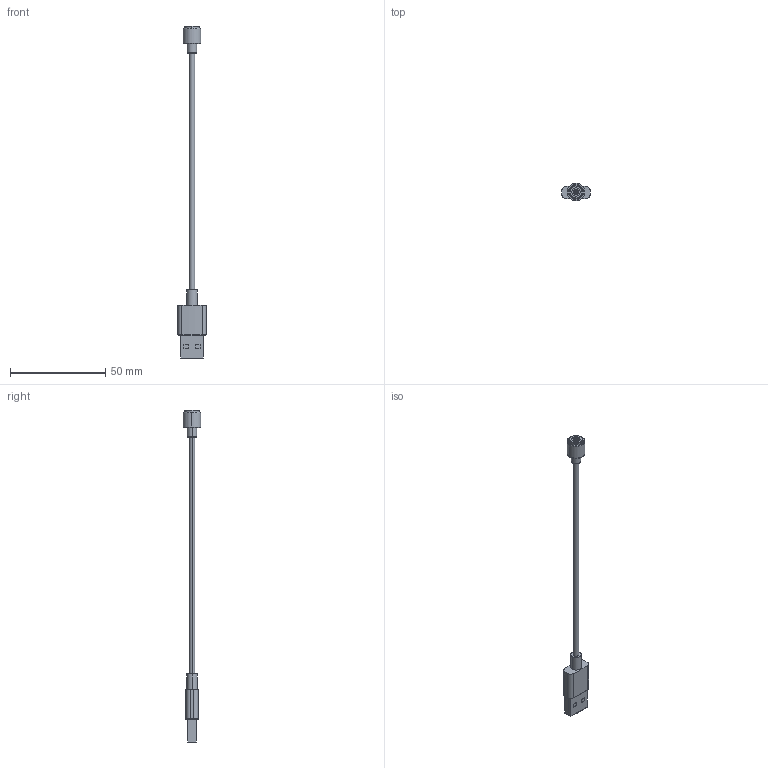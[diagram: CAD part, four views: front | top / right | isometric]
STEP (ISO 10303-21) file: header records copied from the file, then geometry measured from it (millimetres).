
FILE_DESCRIPTION (( 'STEP AP203' ), '1' );
FILE_NAME ('687-C0222A001C00.STEP', '2023-02-09T15:45:17', ( '' ), ( '' ), 'SwSTEP 2.0', 'SolidWorks 2020', '' );
FILE_SCHEMA (( 'CONFIG_CONTROL_DESIGN' ));
Length unit declared in the file: millimetre
Products named in the file (1): 687-C0222A001C00
Bounding box: 14.8 x 9.4 x 174.69 mm (x, y, z)
Surface area: 3758.1 mm2 (no closed solid volume)
Topology: 0 solids, 5 shells, 143 faces, 332 edges, 212 vertices
Faces by surface type: plane 68, cylinder 43, torus 18, bspline 10, cone 2, sphere 2
Entity records: 4375 total; most frequent: CARTESIAN_POINT 1015, DIRECTION 697, ORIENTED_EDGE 660, EDGE_CURVE 332, AXIS2_PLACEMENT_3D 260, VERTEX_POINT 212, VECTOR 177, LINE 177
